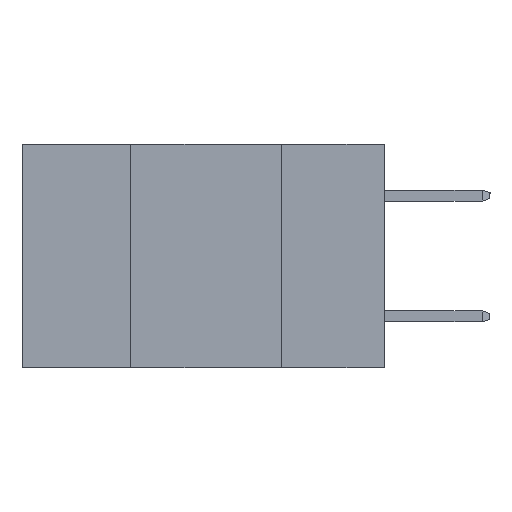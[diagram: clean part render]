
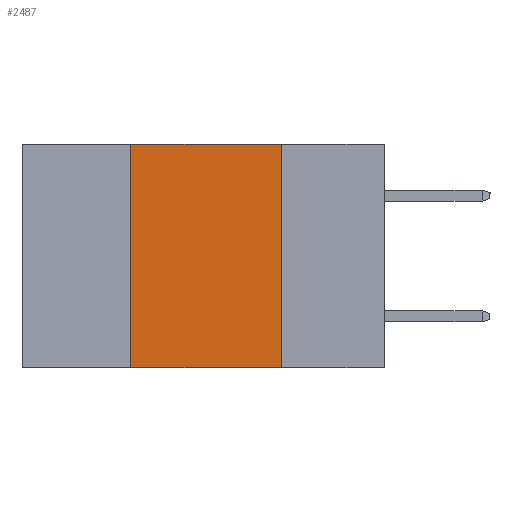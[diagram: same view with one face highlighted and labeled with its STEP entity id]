
A CAD part, left-side view. The second image highlights one B-rep face of the part: STEP entity #2487.
In plain terms, the highlighted planar face has unit normal (-1, 0, 0).
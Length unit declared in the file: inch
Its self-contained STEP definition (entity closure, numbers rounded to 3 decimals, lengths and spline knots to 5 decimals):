
#771 = LINE ( 'NONE', #8453, #5432 ) ;
#2285 = LINE ( 'NONE', #23531, #13219 ) ;
#2487 = ADVANCED_FACE ( 'NONE', ( #19013 ), #5472, .F. ) ;
#2765 = VERTEX_POINT ( 'NONE', #11981 ) ;
#3376 = ORIENTED_EDGE ( 'NONE', *, *, #4686, .F. ) ;
#3831 = DIRECTION ( 'NONE',  ( 1., 0., 0. ) ) ;
#4251 = EDGE_CURVE ( 'NONE', #14803, #9393, #771, .T. ) ;
#4686 = EDGE_CURVE ( 'NONE', #2765, #17071, #14338, .T. ) ;
#4796 = CARTESIAN_POINT ( 'NONE',  ( 0., 0.42, -0.37 ) ) ;
#5253 = DIRECTION ( 'NONE',  ( 0., -1., 0. ) ) ;
#5432 = VECTOR ( 'NONE', #16135, 39.37008 ) ;
#5472 = PLANE ( 'NONE',  #23716 ) ;
#6800 = ORIENTED_EDGE ( 'NONE', *, *, #4251, .F. ) ;
#7140 = CARTESIAN_POINT ( 'NONE',  ( 0., 0.42, 0. ) ) ;
#7901 = CARTESIAN_POINT ( 'NONE',  ( 0., 0.17, -0.37 ) ) ;
#8453 = CARTESIAN_POINT ( 'NONE',  ( 0., 0.17, -0.37 ) ) ;
#9299 = EDGE_LOOP ( 'NONE', ( #6800, #13103, #3376, #22504 ) ) ;
#9393 = VERTEX_POINT ( 'NONE', #7901 ) ;
#10206 = DIRECTION ( 'NONE',  ( 0., -1., 0. ) ) ;
#10696 = VECTOR ( 'NONE', #12464, 39.37008 ) ;
#11045 = EDGE_CURVE ( 'NONE', #17071, #14803, #15167, .T. ) ;
#11981 = CARTESIAN_POINT ( 'NONE',  ( 0., 0.42, -0.37 ) ) ;
#12464 = DIRECTION ( 'NONE',  ( 0., 0., 1. ) ) ;
#13103 = ORIENTED_EDGE ( 'NONE', *, *, #11045, .F. ) ;
#13219 = VECTOR ( 'NONE', #10206, 39.37008 ) ;
#13260 = CARTESIAN_POINT ( 'NONE',  ( 0., 0.6, 0. ) ) ;
#14338 = LINE ( 'NONE', #4796, #10696 ) ;
#14803 = VERTEX_POINT ( 'NONE', #17173 ) ;
#15167 = LINE ( 'NONE', #22837, #19390 ) ;
#16135 = DIRECTION ( 'NONE',  ( 0., 0., -1. ) ) ;
#16789 = DIRECTION ( 'NONE',  ( 0., 0., -1. ) ) ;
#17071 = VERTEX_POINT ( 'NONE', #7140 ) ;
#17173 = CARTESIAN_POINT ( 'NONE',  ( 0., 0.17, 0. ) ) ;
#19013 = FACE_OUTER_BOUND ( 'NONE', #9299, .T. ) ;
#19390 = VECTOR ( 'NONE', #5253, 39.37008 ) ;
#19655 = EDGE_CURVE ( 'NONE', #2765, #9393, #2285, .T. ) ;
#22504 = ORIENTED_EDGE ( 'NONE', *, *, #19655, .T. ) ;
#22837 = CARTESIAN_POINT ( 'NONE',  ( 0., 0.6, 0. ) ) ;
#23531 = CARTESIAN_POINT ( 'NONE',  ( 0., 0.6, -0.37 ) ) ;
#23716 = AXIS2_PLACEMENT_3D ( 'NONE', #13260, #3831, #16789 ) ;
